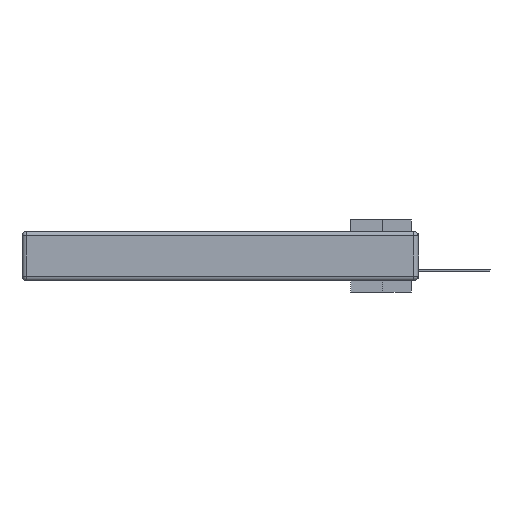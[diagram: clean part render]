
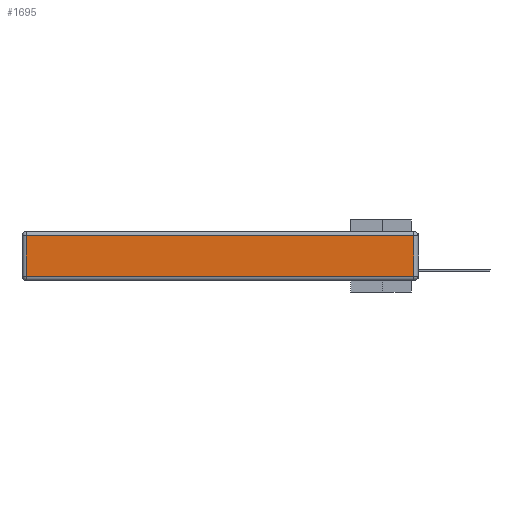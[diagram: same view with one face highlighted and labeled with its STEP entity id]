
A CAD part, left-side view. The second image highlights one B-rep face of the part: STEP entity #1695.
In plain terms, the highlighted planar face has unit normal (-1, 0, 0).
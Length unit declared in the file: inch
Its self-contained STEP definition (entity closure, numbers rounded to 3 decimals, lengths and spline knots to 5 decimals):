
#4 = PLANE ( 'NONE',  #13808 ) ;
#161 = DIRECTION ( 'NONE',  ( 0., 0., 1. ) ) ;
#325 = CARTESIAN_POINT ( 'NONE',  ( 0., 0., -0.343 ) ) ;
#640 = LINE ( 'NONE', #25010, #4070 ) ;
#1695 = ADVANCED_FACE ( 'NONE', ( #27660 ), #4, .T. ) ;
#2298 = VECTOR ( 'NONE', #24683, 39.37008 ) ;
#2584 = ORIENTED_EDGE ( 'NONE', *, *, #13821, .T. ) ;
#3663 = CARTESIAN_POINT ( 'NONE',  ( 0., 0.03, -0.313 ) ) ;
#4070 = VECTOR ( 'NONE', #30251, 39.37008 ) ;
#5196 = VERTEX_POINT ( 'NONE', #3663 ) ;
#5280 = LINE ( 'NONE', #12565, #13239 ) ;
#5555 = DIRECTION ( 'NONE',  ( -1., 0., 0. ) ) ;
#6337 = VERTEX_POINT ( 'NONE', #17080 ) ;
#8320 = CARTESIAN_POINT ( 'NONE',  ( 0., 0.03, -0.343 ) ) ;
#8812 = LINE ( 'NONE', #8320, #21738 ) ;
#10013 = EDGE_CURVE ( 'NONE', #25821, #17907, #5280, .T. ) ;
#11872 = LINE ( 'NONE', #31545, #2298 ) ;
#12565 = CARTESIAN_POINT ( 'NONE',  ( 0., 2.72, -0.343 ) ) ;
#13197 = DIRECTION ( 'NONE',  ( 0., 0., 1. ) ) ;
#13239 = VECTOR ( 'NONE', #30476, 39.37008 ) ;
#13551 = EDGE_CURVE ( 'NONE', #17907, #5196, #640, .T. ) ;
#13707 = ORIENTED_EDGE ( 'NONE', *, *, #10013, .T. ) ;
#13808 = AXIS2_PLACEMENT_3D ( 'NONE', #325, #5555, #161 ) ;
#13821 = EDGE_CURVE ( 'NONE', #6337, #25821, #11872, .T. ) ;
#17080 = CARTESIAN_POINT ( 'NONE',  ( 0., 0.03, -0.03 ) ) ;
#17907 = VERTEX_POINT ( 'NONE', #30144 ) ;
#18491 = EDGE_CURVE ( 'NONE', #5196, #6337, #8812, .T. ) ;
#20422 = ORIENTED_EDGE ( 'NONE', *, *, #18491, .T. ) ;
#21738 = VECTOR ( 'NONE', #13197, 39.37008 ) ;
#23477 = EDGE_LOOP ( 'NONE', ( #27334, #20422, #2584, #13707 ) ) ;
#24683 = DIRECTION ( 'NONE',  ( 0., 1., 0. ) ) ;
#25010 = CARTESIAN_POINT ( 'NONE',  ( 0., 0., -0.313 ) ) ;
#25821 = VERTEX_POINT ( 'NONE', #29054 ) ;
#27334 = ORIENTED_EDGE ( 'NONE', *, *, #13551, .T. ) ;
#27660 = FACE_OUTER_BOUND ( 'NONE', #23477, .T. ) ;
#29054 = CARTESIAN_POINT ( 'NONE',  ( 0., 2.72, -0.03 ) ) ;
#30144 = CARTESIAN_POINT ( 'NONE',  ( 0., 2.72, -0.313 ) ) ;
#30251 = DIRECTION ( 'NONE',  ( 0., -1., 0. ) ) ;
#30476 = DIRECTION ( 'NONE',  ( 0., 0., -1. ) ) ;
#31545 = CARTESIAN_POINT ( 'NONE',  ( 0., 2.75, -0.03 ) ) ;
